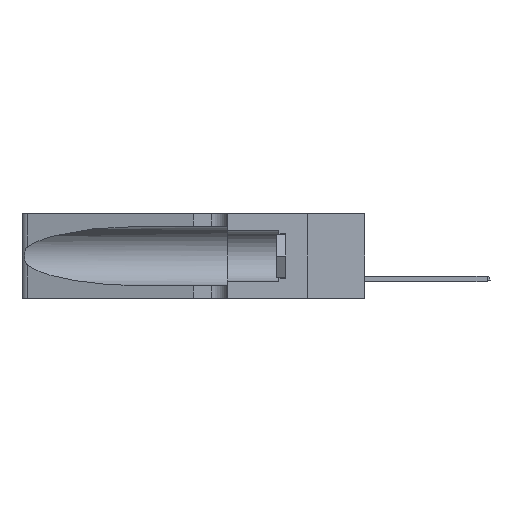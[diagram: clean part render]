
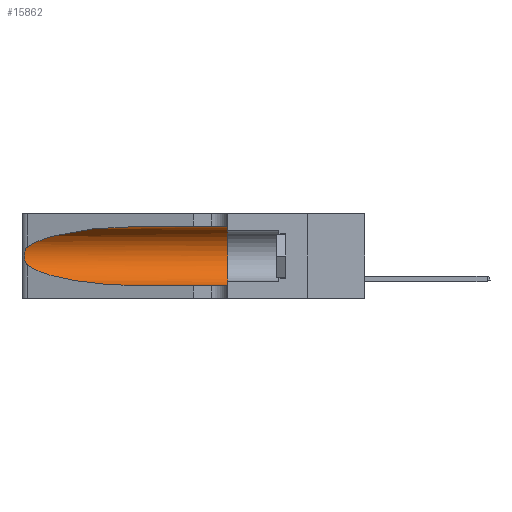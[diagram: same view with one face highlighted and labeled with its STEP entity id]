
A CAD part, left-side view. The second image highlights one B-rep face of the part: STEP entity #15862.
In plain terms, the highlighted cylindrical face has radius 3.308 mm (diameter 6.617 mm), a partial arc.
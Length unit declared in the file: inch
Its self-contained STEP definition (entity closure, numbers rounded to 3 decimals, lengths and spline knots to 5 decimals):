
#159 = CARTESIAN_POINT ( 'NONE',  ( 0.25787, 1.23484, 0.2124 ) ) ;
#830 = CARTESIAN_POINT ( 'NONE',  ( 0.2373, 1.15595, 0.28018 ) ) ;
#1059 = CARTESIAN_POINT ( 'NONE',  ( 0.18966, 0.96281, 0.31525 ) ) ;
#1340 = DIRECTION ( 'NONE',  ( 0., -1., 0. ) ) ;
#1500 = DIRECTION ( 'NONE',  ( 0., 1., 0. ) ) ;
#2018 = CARTESIAN_POINT ( 'NONE',  ( 0.25639, 1.23184, 0.21858 ) ) ;
#2029 = CARTESIAN_POINT ( 'NONE',  ( 0.25487, 1.22718, 0.14631 ) ) ;
#2389 = LINE ( 'NONE', #5048, #9738 ) ;
#2405 = AXIS2_PLACEMENT_3D ( 'NONE', #10323, #4999, #10429 ) ;
#3380 = ORIENTED_EDGE ( 'NONE', *, *, #24933, .F. ) ;
#3638 = CARTESIAN_POINT ( 'NONE',  ( 0.25487, 1.22718, 0.22369 ) ) ;
#3964 = CARTESIAN_POINT ( 'NONE',  ( 0.18966, 0.96281, 0.05475 ) ) ;
#4908 = CARTESIAN_POINT ( 'NONE',  ( 0.26075, 1.23896, 0.178 ) ) ;
#4999 = DIRECTION ( 'NONE',  ( 0., -1., 0. ) ) ;
#5017 = CARTESIAN_POINT ( 'NONE',  ( 0.25789, 1.23486, 0.15765 ) ) ;
#5048 = CARTESIAN_POINT ( 'NONE',  ( 0.1305, 1.61858, 0.05475 ) ) ;
#5927 = CARTESIAN_POINT ( 'NONE',  ( 0.25487, 1.22718, 0.22369 ) ) ;
#6431 = CARTESIAN_POINT ( 'NONE',  ( 0.1305, 1.61858, 0.31525 ) ) ;
#7689 = CARTESIAN_POINT ( 'NONE',  ( 0.26075, 1.23896, 0.19203 ) ) ;
#7904 = CARTESIAN_POINT ( 'NONE',  ( 0.25856, 1.23593, 0.16098 ) ) ;
#7987 = B_SPLINE_CURVE_WITH_KNOTS ( 'NONE', 3,
 ( #5927, #12401, #2018, #159, #15677, #20726, #7689, #4908, #12831, #7904, #5017, #10556, #28796, #12943 ),
 .UNSPECIFIED., .F., .F.,
 ( 4, 2, 2, 2, 2, 2, 4 ),
 ( 0., 0.00027, 0.00053, 0.00107, 0.0016, 0.00187, 0.00214 ),
 .UNSPECIFIED. ) ;
#8755 = VECTOR ( 'NONE', #1340, 39.37008 ) ;
#9738 = VECTOR ( 'NONE', #33629, 39.37008 ) ;
#10156 = VERTEX_POINT ( 'NONE', #17903 ) ;
#10323 = CARTESIAN_POINT ( 'NONE',  ( 0.1305, 1.61858, 0.185 ) ) ;
#10379 = ORIENTED_EDGE ( 'NONE', *, *, #23754, .T. ) ;
#10429 = DIRECTION ( 'NONE',  ( 0., 0., -1. ) ) ;
#10556 = CARTESIAN_POINT ( 'NONE',  ( 0.25639, 1.23186, 0.15144 ) ) ;
#11773 = CARTESIAN_POINT ( 'NONE',  ( 0.1305, 0.35, 0.185 ) ) ;
#12401 = CARTESIAN_POINT ( 'NONE',  ( 0.25555, 1.22994, 0.2215 ) ) ;
#12831 = CARTESIAN_POINT ( 'NONE',  ( 0.26017, 1.23833, 0.17102 ) ) ;
#12943 = CARTESIAN_POINT ( 'NONE',  ( 0.25487, 1.22718, 0.14631 ) ) ;
#13780 = VERTEX_POINT ( 'NONE', #21775 ) ;
#13919 = CARTESIAN_POINT ( 'NONE',  ( 0.1305, 0.72297, 0.31525 ) ) ;
#14884 = LINE ( 'NONE', #6431, #8755 ) ;
#15677 = CARTESIAN_POINT ( 'NONE',  ( 0.25854, 1.2359, 0.20912 ) ) ;
#15862 = ADVANCED_FACE ( 'NONE', ( #30413 ), #26339, .F. ) ;
#16949 = CARTESIAN_POINT ( 'NONE',  ( 0.1305, 0.35, 0.05475 ) ) ;
#17131 = ORIENTED_EDGE ( 'NONE', *, *, #20430, .F. ) ;
#17903 = CARTESIAN_POINT ( 'NONE',  ( 0.1305, 0.72297, 0.31525 ) ) ;
#18756 = EDGE_CURVE ( 'NONE', #13780, #25747, #2389, .T. ) ;
#19470 = VERTEX_POINT ( 'NONE', #31012 ) ;
#19740 =( BOUNDED_CURVE ( )  B_SPLINE_CURVE ( 3, ( #30226, #22588, #3964, #30455 ),
 .UNSPECIFIED., .F., .T. ) 
 B_SPLINE_CURVE_WITH_KNOTS ( ( 4, 4 ),
 ( 3.44316, 4.71239 ),
 .UNSPECIFIED. ) 
 CURVE ( )  GEOMETRIC_REPRESENTATION_ITEM ( )  RATIONAL_B_SPLINE_CURVE ( ( 1., 0.87, 0.87, 1. ) ) 
 REPRESENTATION_ITEM ( '' )  );
#20430 = EDGE_CURVE ( 'NONE', #26079, #25747, #20659, .T. ) ;
#20659 = CIRCLE ( 'NONE', #30690, 0.13025 ) ;
#20726 = CARTESIAN_POINT ( 'NONE',  ( 0.26018, 1.23835, 0.19895 ) ) ;
#21775 = CARTESIAN_POINT ( 'NONE',  ( 0.1305, 0.72297, 0.05475 ) ) ;
#22583 = VERTEX_POINT ( 'NONE', #2029 ) ;
#22588 = CARTESIAN_POINT ( 'NONE',  ( 0.2373, 1.15595, 0.08982 ) ) ;
#23754 = EDGE_CURVE ( 'NONE', #19470, #22583, #7987, .T. ) ;
#24406 = EDGE_LOOP ( 'NONE', ( #31588, #10379, #27964, #28619, #17131, #3380 ) ) ;
#24933 = EDGE_CURVE ( 'NONE', #10156, #26079, #14884, .T. ) ;
#25747 = VERTEX_POINT ( 'NONE', #16949 ) ;
#26079 = VERTEX_POINT ( 'NONE', #27296 ) ;
#26339 = CYLINDRICAL_SURFACE ( 'NONE', #2405, 0.13025 ) ;
#27296 = CARTESIAN_POINT ( 'NONE',  ( 0.1305, 0.35, 0.31525 ) ) ;
#27628 = DIRECTION ( 'NONE',  ( 0., 0., 1. ) ) ;
#27964 = ORIENTED_EDGE ( 'NONE', *, *, #30094, .T. ) ;
#28306 =( BOUNDED_CURVE ( )  B_SPLINE_CURVE ( 3, ( #13919, #1059, #830, #3638 ),
 .UNSPECIFIED., .F., .F. ) 
 B_SPLINE_CURVE_WITH_KNOTS ( ( 4, 4 ),
 ( 1.5708, 2.84003 ),
 .UNSPECIFIED. ) 
 CURVE ( )  GEOMETRIC_REPRESENTATION_ITEM ( )  RATIONAL_B_SPLINE_CURVE ( ( 1., 0.87, 0.87, 1. ) ) 
 REPRESENTATION_ITEM ( '' )  );
#28619 = ORIENTED_EDGE ( 'NONE', *, *, #18756, .T. ) ;
#28730 = EDGE_CURVE ( 'NONE', #10156, #19470, #28306, .T. ) ;
#28796 = CARTESIAN_POINT ( 'NONE',  ( 0.25555, 1.22993, 0.14849 ) ) ;
#30094 = EDGE_CURVE ( 'NONE', #22583, #13780, #19740, .T. ) ;
#30226 = CARTESIAN_POINT ( 'NONE',  ( 0.25487, 1.22718, 0.14631 ) ) ;
#30413 = FACE_OUTER_BOUND ( 'NONE', #24406, .T. ) ;
#30455 = CARTESIAN_POINT ( 'NONE',  ( 0.1305, 0.72297, 0.05475 ) ) ;
#30690 = AXIS2_PLACEMENT_3D ( 'NONE', #11773, #1500, #27628 ) ;
#31012 = CARTESIAN_POINT ( 'NONE',  ( 0.25487, 1.22718, 0.22369 ) ) ;
#31588 = ORIENTED_EDGE ( 'NONE', *, *, #28730, .T. ) ;
#33629 = DIRECTION ( 'NONE',  ( 0., -1., 0. ) ) ;
